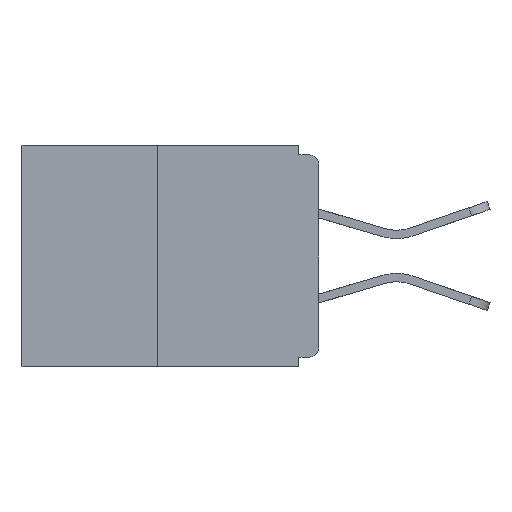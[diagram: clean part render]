
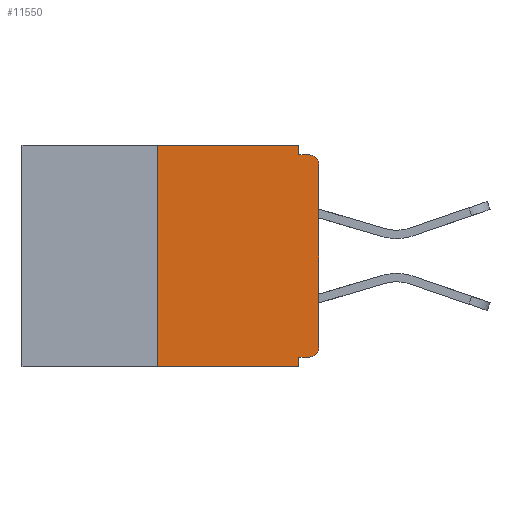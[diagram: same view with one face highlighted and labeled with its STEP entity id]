
A CAD part, left-side view. The second image highlights one B-rep face of the part: STEP entity #11550.
In plain terms, the highlighted planar face has unit normal (-1, 0, 0).
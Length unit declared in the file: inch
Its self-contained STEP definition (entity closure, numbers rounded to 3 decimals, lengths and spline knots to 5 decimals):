
#189 = CARTESIAN_POINT ( 'NONE',  ( 0., 0., -0.03 ) ) ;
#198 = DIRECTION ( 'NONE',  ( 0., 0., 1. ) ) ;
#458 = VERTEX_POINT ( 'NONE', #12735 ) ;
#506 = AXIS2_PLACEMENT_3D ( 'NONE', #17173, #13770, #872 ) ;
#663 = CARTESIAN_POINT ( 'NONE',  ( 0., 0.25, 0. ) ) ;
#821 = EDGE_CURVE ( 'NONE', #2353, #14587, #14277, .T. ) ;
#872 = DIRECTION ( 'NONE',  ( 0., 0., -1. ) ) ;
#1157 = DIRECTION ( 'NONE',  ( 0., 0., -1. ) ) ;
#1278 = CARTESIAN_POINT ( 'NONE',  ( 0., 0.031, -0.328 ) ) ;
#1682 = VERTEX_POINT ( 'NONE', #663 ) ;
#1699 = VECTOR ( 'NONE', #10048, 39.37008 ) ;
#1735 = DIRECTION ( 'NONE',  ( 0., 0., 1. ) ) ;
#1738 = VECTOR ( 'NONE', #1157, 39.37008 ) ;
#2078 = DIRECTION ( 'NONE',  ( 0., 1., 0. ) ) ;
#2353 = VERTEX_POINT ( 'NONE', #6234 ) ;
#2378 = VERTEX_POINT ( 'NONE', #11123 ) ;
#2701 = DIRECTION ( 'NONE',  ( 0., 0., -1. ) ) ;
#2959 = LINE ( 'NONE', #11699, #1699 ) ;
#3414 = VECTOR ( 'NONE', #17206, 39.37008 ) ;
#4150 = ORIENTED_EDGE ( 'NONE', *, *, #5626, .T. ) ;
#4282 = VECTOR ( 'NONE', #13922, 39.37008 ) ;
#4939 = VECTOR ( 'NONE', #2078, 39.37008 ) ;
#5082 = LINE ( 'NONE', #13785, #4282 ) ;
#5395 = ORIENTED_EDGE ( 'NONE', *, *, #18064, .F. ) ;
#5490 = VERTEX_POINT ( 'NONE', #189 ) ;
#5626 = EDGE_CURVE ( 'NONE', #5704, #16621, #5082, .T. ) ;
#5704 = VERTEX_POINT ( 'NONE', #10106 ) ;
#5750 = CARTESIAN_POINT ( 'NONE',  ( 0., 0.031, 0. ) ) ;
#6000 = CARTESIAN_POINT ( 'NONE',  ( 0., 0.031, -0.343 ) ) ;
#6221 = DIRECTION ( 'NONE',  ( 0., -1., 0. ) ) ;
#6234 = CARTESIAN_POINT ( 'NONE',  ( 0., 0.015, -0.328 ) ) ;
#6922 = AXIS2_PLACEMENT_3D ( 'NONE', #7550, #9202, #2701 ) ;
#7082 = LINE ( 'NONE', #9557, #12728 ) ;
#7284 = AXIS2_PLACEMENT_3D ( 'NONE', #19315, #9350, #14150 ) ;
#7550 = CARTESIAN_POINT ( 'NONE',  ( 0., 0.015, -0.313 ) ) ;
#7905 = EDGE_CURVE ( 'NONE', #5704, #1682, #12369, .T. ) ;
#8010 = VECTOR ( 'NONE', #1735, 39.37008 ) ;
#8177 = ORIENTED_EDGE ( 'NONE', *, *, #9015, .T. ) ;
#8463 = CARTESIAN_POINT ( 'NONE',  ( 0., 0.031, -0.343 ) ) ;
#9015 = EDGE_CURVE ( 'NONE', #5490, #13534, #15919, .T. ) ;
#9202 = DIRECTION ( 'NONE',  ( -1., 0., 0. ) ) ;
#9350 = DIRECTION ( 'NONE',  ( -1., 0., 0. ) ) ;
#9557 = CARTESIAN_POINT ( 'NONE',  ( 0., 0.46, 0. ) ) ;
#9779 = LINE ( 'NONE', #18327, #4939 ) ;
#9807 = LINE ( 'NONE', #5750, #3414 ) ;
#10048 = DIRECTION ( 'NONE',  ( 0., -1., 0. ) ) ;
#10106 = CARTESIAN_POINT ( 'NONE',  ( 0., 0.25, -0.343 ) ) ;
#10590 = ORIENTED_EDGE ( 'NONE', *, *, #18649, .T. ) ;
#11123 = CARTESIAN_POINT ( 'NONE',  ( 0., 0.031, -0.015 ) ) ;
#11550 = ADVANCED_FACE ( 'NONE', ( #20006 ), #13909, .F. ) ;
#11657 = EDGE_CURVE ( 'NONE', #12062, #16621, #17925, .T. ) ;
#11699 = CARTESIAN_POINT ( 'NONE',  ( 0., 0., -0.015 ) ) ;
#11893 = CARTESIAN_POINT ( 'NONE',  ( 0., 0., 0. ) ) ;
#12062 = VERTEX_POINT ( 'NONE', #1278 ) ;
#12369 = LINE ( 'NONE', #16315, #8010 ) ;
#12728 = VECTOR ( 'NONE', #6221, 39.37008 ) ;
#12735 = CARTESIAN_POINT ( 'NONE',  ( 0., 0.031, 0. ) ) ;
#12865 = ORIENTED_EDGE ( 'NONE', *, *, #16035, .F. ) ;
#13534 = VERTEX_POINT ( 'NONE', #16548 ) ;
#13770 = DIRECTION ( 'NONE',  ( 1., 0., 0. ) ) ;
#13785 = CARTESIAN_POINT ( 'NONE',  ( 0., 0.46, -0.343 ) ) ;
#13864 = EDGE_CURVE ( 'NONE', #2378, #13534, #2959, .T. ) ;
#13909 = PLANE ( 'NONE',  #506 ) ;
#13922 = DIRECTION ( 'NONE',  ( 0., -1., 0. ) ) ;
#14150 = DIRECTION ( 'NONE',  ( 0., 0., -1. ) ) ;
#14277 = CIRCLE ( 'NONE', #6922, 0.015 ) ;
#14587 = VERTEX_POINT ( 'NONE', #18951 ) ;
#15919 = CIRCLE ( 'NONE', #7284, 0.015 ) ;
#16035 = EDGE_CURVE ( 'NONE', #2353, #12062, #9779, .T. ) ;
#16215 = EDGE_LOOP ( 'NONE', ( #5395, #19242, #4150, #18458, #12865, #17024, #10590, #8177, #20269, #19761 ) ) ;
#16315 = CARTESIAN_POINT ( 'NONE',  ( 0., 0.25, 0. ) ) ;
#16548 = CARTESIAN_POINT ( 'NONE',  ( 0., 0.015, -0.015 ) ) ;
#16621 = VERTEX_POINT ( 'NONE', #8463 ) ;
#16812 = VECTOR ( 'NONE', #198, 39.37008 ) ;
#17024 = ORIENTED_EDGE ( 'NONE', *, *, #821, .T. ) ;
#17173 = CARTESIAN_POINT ( 'NONE',  ( 0., 0.46, 0. ) ) ;
#17206 = DIRECTION ( 'NONE',  ( 0., 0., -1. ) ) ;
#17925 = LINE ( 'NONE', #6000, #1738 ) ;
#18064 = EDGE_CURVE ( 'NONE', #1682, #458, #7082, .T. ) ;
#18155 = LINE ( 'NONE', #11893, #16812 ) ;
#18327 = CARTESIAN_POINT ( 'NONE',  ( 0., 0., -0.328 ) ) ;
#18458 = ORIENTED_EDGE ( 'NONE', *, *, #11657, .F. ) ;
#18649 = EDGE_CURVE ( 'NONE', #14587, #5490, #18155, .T. ) ;
#18951 = CARTESIAN_POINT ( 'NONE',  ( 0., 0., -0.313 ) ) ;
#19242 = ORIENTED_EDGE ( 'NONE', *, *, #7905, .F. ) ;
#19315 = CARTESIAN_POINT ( 'NONE',  ( 0., 0.015, -0.03 ) ) ;
#19761 = ORIENTED_EDGE ( 'NONE', *, *, #21137, .F. ) ;
#20006 = FACE_OUTER_BOUND ( 'NONE', #16215, .T. ) ;
#20269 = ORIENTED_EDGE ( 'NONE', *, *, #13864, .F. ) ;
#21137 = EDGE_CURVE ( 'NONE', #458, #2378, #9807, .T. ) ;
